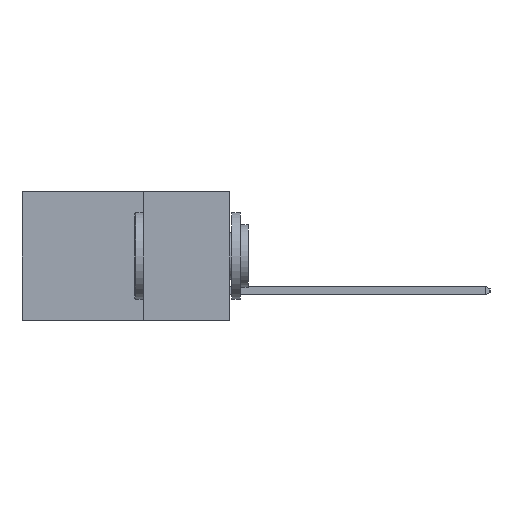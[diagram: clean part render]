
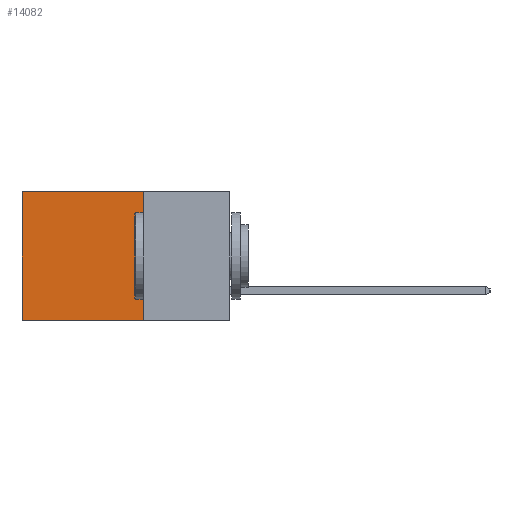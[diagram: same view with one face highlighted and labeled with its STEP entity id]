
A CAD part, left-side view. The second image highlights one B-rep face of the part: STEP entity #14082.
In plain terms, the highlighted planar face has unit normal (-1, 0, 0).
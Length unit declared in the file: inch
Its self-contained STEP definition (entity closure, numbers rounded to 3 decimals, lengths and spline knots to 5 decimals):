
#1345 = LINE ( 'NONE', #7619, #8593 ) ;
#1442 = CARTESIAN_POINT ( 'NONE',  ( 0.2615, 0.6, -0.37 ) ) ;
#1539 = DIRECTION ( 'NONE',  ( 0., 0., -1. ) ) ;
#1914 = ORIENTED_EDGE ( 'NONE', *, *, #17288, .F. ) ;
#2300 = LINE ( 'NONE', #18577, #18515 ) ;
#3103 = EDGE_CURVE ( 'NONE', #17454, #5717, #8446, .T. ) ;
#3433 = AXIS2_PLACEMENT_3D ( 'NONE', #6029, #5993, #5947 ) ;
#3951 = VECTOR ( 'NONE', #13802, 39.37008 ) ;
#4404 = EDGE_LOOP ( 'NONE', ( #13750, #6663, #1914, #10424 ) ) ;
#4713 = CARTESIAN_POINT ( 'NONE',  ( 0.2615, 0.25, -0.37 ) ) ;
#5717 = VERTEX_POINT ( 'NONE', #16822 ) ;
#5947 = DIRECTION ( 'NONE',  ( 0., 0., -1. ) ) ;
#5993 = DIRECTION ( 'NONE',  ( 1., 0., 0. ) ) ;
#6029 = CARTESIAN_POINT ( 'NONE',  ( 0.2615, 0.25, -0.37 ) ) ;
#6055 = PLANE ( 'NONE',  #3433 ) ;
#6663 = ORIENTED_EDGE ( 'NONE', *, *, #17733, .F. ) ;
#7529 = CARTESIAN_POINT ( 'NONE',  ( 0.2615, 0.25, -0.37 ) ) ;
#7619 = CARTESIAN_POINT ( 'NONE',  ( 0.2615, 0.25, -0.37 ) ) ;
#8094 = LINE ( 'NONE', #7529, #3951 ) ;
#8446 = LINE ( 'NONE', #15141, #12093 ) ;
#8593 = VECTOR ( 'NONE', #1539, 39.37008 ) ;
#8904 = FACE_OUTER_BOUND ( 'NONE', #4404, .T. ) ;
#9470 = VERTEX_POINT ( 'NONE', #1442 ) ;
#9574 = DIRECTION ( 'NONE',  ( 0., 0., -1. ) ) ;
#10424 = ORIENTED_EDGE ( 'NONE', *, *, #3103, .T. ) ;
#12093 = VECTOR ( 'NONE', #15078, 39.37008 ) ;
#12284 = VERTEX_POINT ( 'NONE', #4713 ) ;
#13750 = ORIENTED_EDGE ( 'NONE', *, *, #16117, .T. ) ;
#13802 = DIRECTION ( 'NONE',  ( 0., 1., 0. ) ) ;
#14082 = ADVANCED_FACE ( 'NONE', ( #8904 ), #6055, .F. ) ;
#15078 = DIRECTION ( 'NONE',  ( 0., 1., 0. ) ) ;
#15141 = CARTESIAN_POINT ( 'NONE',  ( 0.2615, 0.25, 0. ) ) ;
#16117 = EDGE_CURVE ( 'NONE', #5717, #9470, #2300, .T. ) ;
#16183 = CARTESIAN_POINT ( 'NONE',  ( 0.2615, 0.25, 0. ) ) ;
#16822 = CARTESIAN_POINT ( 'NONE',  ( 0.2615, 0.6, 0. ) ) ;
#17288 = EDGE_CURVE ( 'NONE', #17454, #12284, #1345, .T. ) ;
#17454 = VERTEX_POINT ( 'NONE', #16183 ) ;
#17733 = EDGE_CURVE ( 'NONE', #12284, #9470, #8094, .T. ) ;
#18515 = VECTOR ( 'NONE', #9574, 39.37008 ) ;
#18577 = CARTESIAN_POINT ( 'NONE',  ( 0.2615, 0.6, -0.37 ) ) ;
